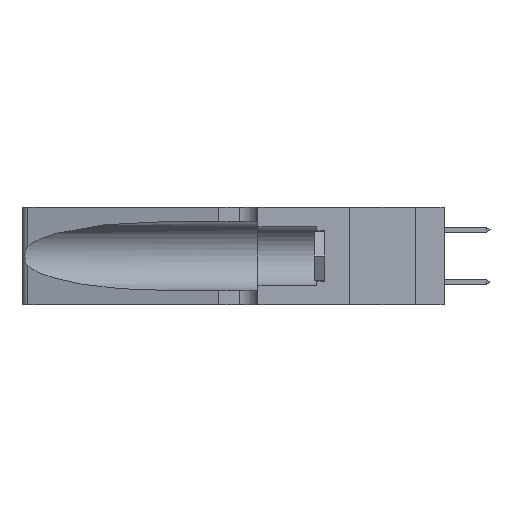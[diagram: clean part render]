
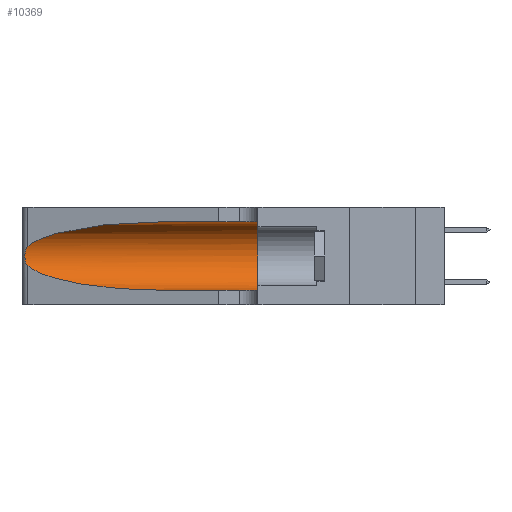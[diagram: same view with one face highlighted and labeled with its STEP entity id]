
A CAD part, left-side view. The second image highlights one B-rep face of the part: STEP entity #10369.
In plain terms, the highlighted cylindrical face has radius 3.308 mm (diameter 6.617 mm), a partial arc.
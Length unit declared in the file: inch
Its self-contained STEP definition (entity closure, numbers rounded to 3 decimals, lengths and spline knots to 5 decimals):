
#374 = CIRCLE ( 'NONE', #15267, 0.13025 ) ;
#607 = CARTESIAN_POINT ( 'NONE',  ( 0.25856, 1.23593, 0.16098 ) ) ;
#772 = CARTESIAN_POINT ( 'NONE',  ( 0.1305, 0.35, 0.05475 ) ) ;
#980 = VERTEX_POINT ( 'NONE', #15183 ) ;
#2419 = CARTESIAN_POINT ( 'NONE',  ( 0.1305, 0.72297, 0.31525 ) ) ;
#2564 = CARTESIAN_POINT ( 'NONE',  ( 0.25789, 1.23486, 0.15765 ) ) ;
#3134 = VERTEX_POINT ( 'NONE', #16970 ) ;
#3368 = DIRECTION ( 'NONE',  ( 0., 0., 1. ) ) ;
#4498 = CARTESIAN_POINT ( 'NONE',  ( 0.25854, 1.2359, 0.20912 ) ) ;
#4568 = CARTESIAN_POINT ( 'NONE',  ( 0.26075, 1.23896, 0.19203 ) ) ;
#4601 = CARTESIAN_POINT ( 'NONE',  ( 0.1305, 1.61858, 0.185 ) ) ;
#4761 = AXIS2_PLACEMENT_3D ( 'NONE', #4601, #19148, #8544 ) ;
#4940 = ORIENTED_EDGE ( 'NONE', *, *, #18495, .T. ) ;
#5189 = EDGE_CURVE ( 'NONE', #3134, #8911, #374, .T. ) ;
#5989 = ORIENTED_EDGE ( 'NONE', *, *, #5189, .F. ) ;
#7088 = DIRECTION ( 'NONE',  ( 0., -1., 0. ) ) ;
#7285 = ORIENTED_EDGE ( 'NONE', *, *, #19248, .T. ) ;
#8030 = CARTESIAN_POINT ( 'NONE',  ( 0.26017, 1.23833, 0.17102 ) ) ;
#8129 = VERTEX_POINT ( 'NONE', #13006 ) ;
#8162 = CARTESIAN_POINT ( 'NONE',  ( 0.25487, 1.22718, 0.14631 ) ) ;
#8265 = CARTESIAN_POINT ( 'NONE',  ( 0.25555, 1.22993, 0.14849 ) ) ;
#8544 = DIRECTION ( 'NONE',  ( 0., 0., -1. ) ) ;
#8911 = VERTEX_POINT ( 'NONE', #772 ) ;
#10369 = ADVANCED_FACE ( 'NONE', ( #22775 ), #10557, .F. ) ;
#10557 = CYLINDRICAL_SURFACE ( 'NONE', #4761, 0.13025 ) ;
#10558 = CARTESIAN_POINT ( 'NONE',  ( 0.2373, 1.15595, 0.28018 ) ) ;
#11087 = CARTESIAN_POINT ( 'NONE',  ( 0.18966, 0.96281, 0.31525 ) ) ;
#11320 = CARTESIAN_POINT ( 'NONE',  ( 0.25487, 1.22718, 0.22369 ) ) ;
#11691 = CARTESIAN_POINT ( 'NONE',  ( 0.1305, 0.72297, 0.05475 ) ) ;
#11718 = CARTESIAN_POINT ( 'NONE',  ( 0.25487, 1.22718, 0.14631 ) ) ;
#12419 = LINE ( 'NONE', #17838, #23496 ) ;
#12501 = DIRECTION ( 'NONE',  ( 0., 1., 0. ) ) ;
#12521 = ORIENTED_EDGE ( 'NONE', *, *, #18707, .T. ) ;
#13006 = CARTESIAN_POINT ( 'NONE',  ( 0.25487, 1.22718, 0.14631 ) ) ;
#13381 = VERTEX_POINT ( 'NONE', #2419 ) ;
#13442 = CARTESIAN_POINT ( 'NONE',  ( 0.1305, 0.35, 0.185 ) ) ;
#14128 = DIRECTION ( 'NONE',  ( 0., -1., 0. ) ) ;
#14559 = ORIENTED_EDGE ( 'NONE', *, *, #15545, .T. ) ;
#15183 = CARTESIAN_POINT ( 'NONE',  ( 0.1305, 0.72297, 0.05475 ) ) ;
#15267 = AXIS2_PLACEMENT_3D ( 'NONE', #13442, #12501, #3368 ) ;
#15307 = CARTESIAN_POINT ( 'NONE',  ( 0.26075, 1.23896, 0.178 ) ) ;
#15459 = CARTESIAN_POINT ( 'NONE',  ( 0.25639, 1.23184, 0.21858 ) ) ;
#15545 = EDGE_CURVE ( 'NONE', #13381, #22750, #18373, .T. ) ;
#16554 = CARTESIAN_POINT ( 'NONE',  ( 0.25487, 1.22718, 0.22369 ) ) ;
#16970 = CARTESIAN_POINT ( 'NONE',  ( 0.1305, 0.35, 0.31525 ) ) ;
#17078 = CARTESIAN_POINT ( 'NONE',  ( 0.2373, 1.15595, 0.08982 ) ) ;
#17102 =( BOUNDED_CURVE ( )  B_SPLINE_CURVE ( 3, ( #8162, #17078, #22582, #11691 ),
 .UNSPECIFIED., .F., .T. ) 
 B_SPLINE_CURVE_WITH_KNOTS ( ( 4, 4 ),
 ( 3.44316, 4.71239 ),
 .UNSPECIFIED. ) 
 CURVE ( )  GEOMETRIC_REPRESENTATION_ITEM ( )  RATIONAL_B_SPLINE_CURVE ( ( 1., 0.87, 0.87, 1. ) ) 
 REPRESENTATION_ITEM ( '' )  );
#17295 = VECTOR ( 'NONE', #14128, 39.37008 ) ;
#17838 = CARTESIAN_POINT ( 'NONE',  ( 0.1305, 1.61858, 0.31525 ) ) ;
#18373 =( BOUNDED_CURVE ( )  B_SPLINE_CURVE ( 3, ( #23445, #11087, #10558, #16554 ),
 .UNSPECIFIED., .F., .T. ) 
 B_SPLINE_CURVE_WITH_KNOTS ( ( 4, 4 ),
 ( 1.5708, 2.84003 ),
 .UNSPECIFIED. ) 
 CURVE ( )  GEOMETRIC_REPRESENTATION_ITEM ( )  RATIONAL_B_SPLINE_CURVE ( ( 1., 0.87, 0.87, 1. ) ) 
 REPRESENTATION_ITEM ( '' )  );
#18495 = EDGE_CURVE ( 'NONE', #8129, #980, #17102, .T. ) ;
#18707 = EDGE_CURVE ( 'NONE', #980, #8911, #21048, .T. ) ;
#18958 = CARTESIAN_POINT ( 'NONE',  ( 0.25787, 1.23484, 0.2124 ) ) ;
#19042 = CARTESIAN_POINT ( 'NONE',  ( 0.25555, 1.22994, 0.2215 ) ) ;
#19148 = DIRECTION ( 'NONE',  ( 0., -1., 0. ) ) ;
#19204 = CARTESIAN_POINT ( 'NONE',  ( 0.25639, 1.23186, 0.15144 ) ) ;
#19248 = EDGE_CURVE ( 'NONE', #22750, #8129, #23420, .T. ) ;
#19502 = ORIENTED_EDGE ( 'NONE', *, *, #21255, .F. ) ;
#20098 = EDGE_LOOP ( 'NONE', ( #14559, #7285, #4940, #12521, #5989, #19502 ) ) ;
#20722 = CARTESIAN_POINT ( 'NONE',  ( 0.25487, 1.22718, 0.22369 ) ) ;
#20887 = CARTESIAN_POINT ( 'NONE',  ( 0.26018, 1.23835, 0.19895 ) ) ;
#21048 = LINE ( 'NONE', #23021, #17295 ) ;
#21255 = EDGE_CURVE ( 'NONE', #13381, #3134, #12419, .T. ) ;
#22582 = CARTESIAN_POINT ( 'NONE',  ( 0.18966, 0.96281, 0.05475 ) ) ;
#22750 = VERTEX_POINT ( 'NONE', #11320 ) ;
#22775 = FACE_OUTER_BOUND ( 'NONE', #20098, .T. ) ;
#23021 = CARTESIAN_POINT ( 'NONE',  ( 0.1305, 1.61858, 0.05475 ) ) ;
#23420 = B_SPLINE_CURVE_WITH_KNOTS ( 'NONE', 3,
 ( #20722, #19042, #15459, #18958, #4498, #20887, #4568, #15307, #8030, #607, #2564, #19204, #8265, #11718 ),
 .UNSPECIFIED., .F., .F.,
 ( 4, 2, 2, 2, 2, 2, 4 ),
 ( 0., 0.00027, 0.00053, 0.00107, 0.0016, 0.00187, 0.00214 ),
 .UNSPECIFIED. ) ;
#23445 = CARTESIAN_POINT ( 'NONE',  ( 0.1305, 0.72297, 0.31525 ) ) ;
#23496 = VECTOR ( 'NONE', #7088, 39.37008 ) ;
